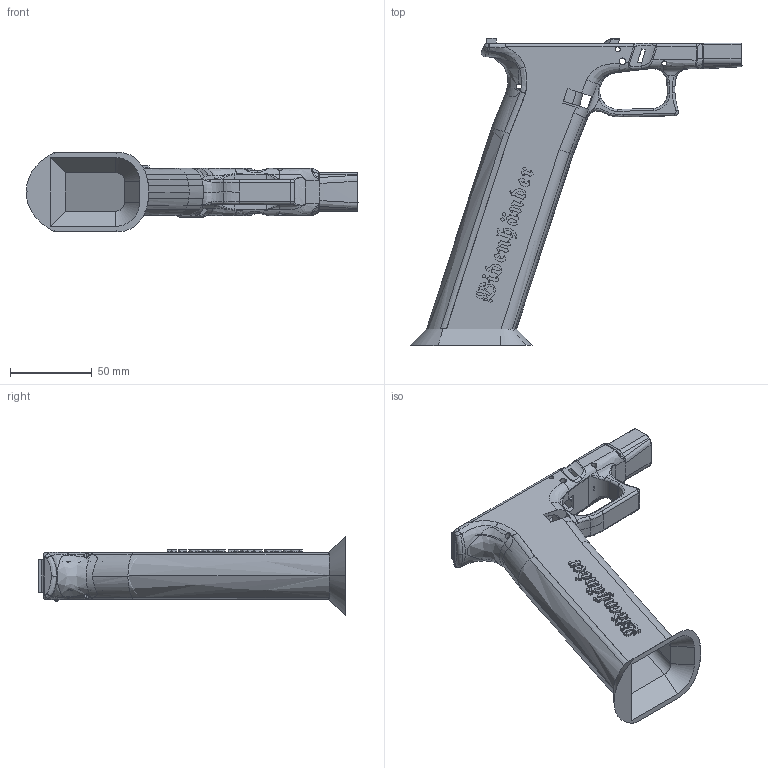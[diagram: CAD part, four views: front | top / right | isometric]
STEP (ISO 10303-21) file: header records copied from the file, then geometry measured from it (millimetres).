
FILE_DESCRIPTION (( 'STEP AP203' ), '1' );
FILE_NAME ('BidenHander.STEP', '2021-04-30T21:56:43', ( '' ), ( '' ), 'SwSTEP 2.0', 'SolidWorks 2019', '' );
FILE_SCHEMA (( 'CONFIG_CONTROL_DESIGN' ));
Length unit declared in the file: millimetre
Products named in the file (1): BidenHander
Bounding box: 202.87 x 187.55 x 48.8 mm (x, y, z)
Volume: 134995.5 mm3; surface area: 69094.9 mm2
Topology: 1 solids, 3 shells, 1163 faces, 3415 edges, 2227 vertices
Faces by surface type: plane 526, bspline 457, cylinder 155, torus 15, cone 10
Entity records: 63569 total; most frequent: CARTESIAN_POINT 36787, ORIENTED_EDGE 6766, DIRECTION 3698, EDGE_CURVE 3383, VERTEX_POINT 2227, VECTOR 1834, LINE 1834, B_SPLINE_CURVE_WITH_KNOTS 1236
